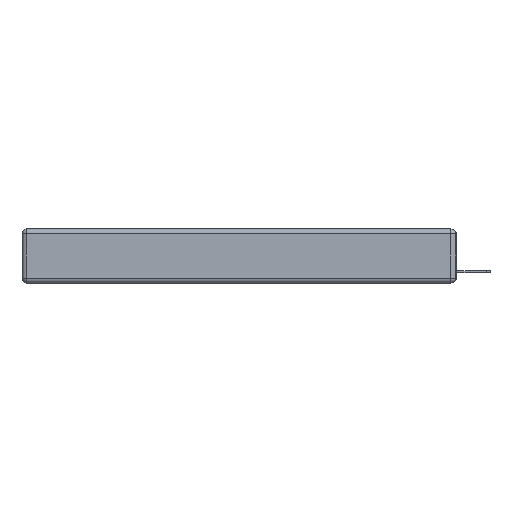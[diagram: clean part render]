
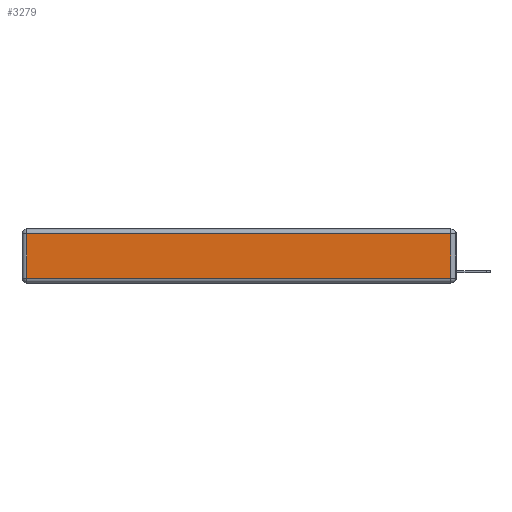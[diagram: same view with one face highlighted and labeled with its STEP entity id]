
A CAD part, left-side view. The second image highlights one B-rep face of the part: STEP entity #3279.
In plain terms, the highlighted planar face has unit normal (-1, 0, 0).
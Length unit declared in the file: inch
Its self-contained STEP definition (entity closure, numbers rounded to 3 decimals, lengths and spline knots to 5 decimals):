
#7 = CARTESIAN_POINT ( 'NONE',  ( 0., 0., -0.343 ) ) ;
#9 = LINE ( 'NONE', #15869, #1159 ) ;
#1159 = VECTOR ( 'NONE', #9673, 39.37008 ) ;
#1771 = LINE ( 'NONE', #9990, #14511 ) ;
#2021 = EDGE_CURVE ( 'NONE', #5865, #13587, #1771, .T. ) ;
#2378 = EDGE_CURVE ( 'NONE', #12776, #5865, #9, .T. ) ;
#2443 = DIRECTION ( 'NONE',  ( 0., 0., 1. ) ) ;
#3159 = ORIENTED_EDGE ( 'NONE', *, *, #2378, .T. ) ;
#3279 = ADVANCED_FACE ( 'NONE', ( #13522 ), #14690, .T. ) ;
#3417 = CARTESIAN_POINT ( 'NONE',  ( 0., 0.03, -0.313 ) ) ;
#3663 = CARTESIAN_POINT ( 'NONE',  ( 0., 2.72, -0.343 ) ) ;
#4094 = ORIENTED_EDGE ( 'NONE', *, *, #2021, .T. ) ;
#5060 = DIRECTION ( 'NONE',  ( -1., 0., 0. ) ) ;
#5282 = VECTOR ( 'NONE', #14699, 39.37008 ) ;
#5865 = VERTEX_POINT ( 'NONE', #6578 ) ;
#6578 = CARTESIAN_POINT ( 'NONE',  ( 0., 0.03, -0.03 ) ) ;
#6606 = VECTOR ( 'NONE', #10879, 39.37008 ) ;
#7480 = ORIENTED_EDGE ( 'NONE', *, *, #15864, .T. ) ;
#7553 = LINE ( 'NONE', #12216, #6606 ) ;
#9537 = AXIS2_PLACEMENT_3D ( 'NONE', #7, #5060, #2443 ) ;
#9673 = DIRECTION ( 'NONE',  ( 0., 0., 1. ) ) ;
#9675 = LINE ( 'NONE', #3663, #5282 ) ;
#9990 = CARTESIAN_POINT ( 'NONE',  ( 0., 2.75, -0.03 ) ) ;
#10055 = DIRECTION ( 'NONE',  ( 0., 1., 0. ) ) ;
#10105 = ORIENTED_EDGE ( 'NONE', *, *, #14076, .T. ) ;
#10626 = VERTEX_POINT ( 'NONE', #15930 ) ;
#10879 = DIRECTION ( 'NONE',  ( 0., -1., 0. ) ) ;
#12216 = CARTESIAN_POINT ( 'NONE',  ( 0., 0., -0.313 ) ) ;
#12685 = CARTESIAN_POINT ( 'NONE',  ( 0., 2.72, -0.03 ) ) ;
#12776 = VERTEX_POINT ( 'NONE', #3417 ) ;
#13522 = FACE_OUTER_BOUND ( 'NONE', #13794, .T. ) ;
#13587 = VERTEX_POINT ( 'NONE', #12685 ) ;
#13794 = EDGE_LOOP ( 'NONE', ( #7480, #3159, #4094, #10105 ) ) ;
#14076 = EDGE_CURVE ( 'NONE', #13587, #10626, #9675, .T. ) ;
#14511 = VECTOR ( 'NONE', #10055, 39.37008 ) ;
#14690 = PLANE ( 'NONE',  #9537 ) ;
#14699 = DIRECTION ( 'NONE',  ( 0., 0., -1. ) ) ;
#15864 = EDGE_CURVE ( 'NONE', #10626, #12776, #7553, .T. ) ;
#15869 = CARTESIAN_POINT ( 'NONE',  ( 0., 0.03, -0.343 ) ) ;
#15930 = CARTESIAN_POINT ( 'NONE',  ( 0., 2.72, -0.313 ) ) ;
